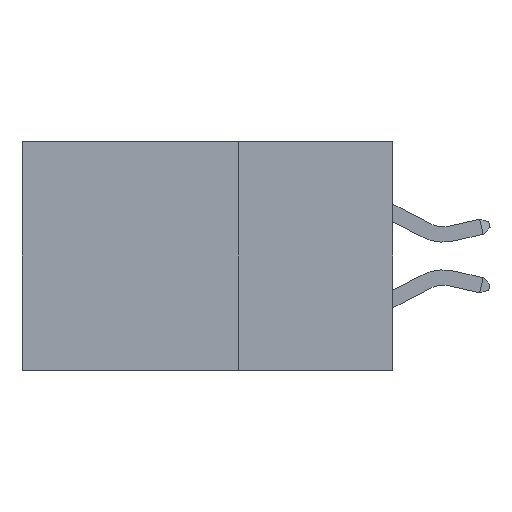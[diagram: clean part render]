
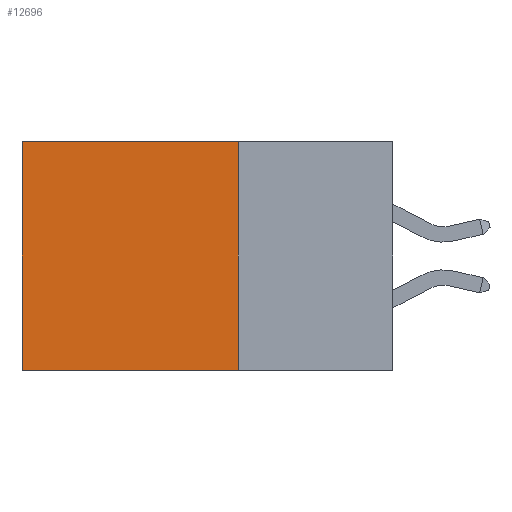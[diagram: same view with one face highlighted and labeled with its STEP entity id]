
A CAD part, left-side view. The second image highlights one B-rep face of the part: STEP entity #12696.
In plain terms, the highlighted planar face has unit normal (-1, 0, 0).
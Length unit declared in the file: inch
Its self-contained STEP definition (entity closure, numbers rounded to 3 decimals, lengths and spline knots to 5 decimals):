
#2719 = AXIS2_PLACEMENT_3D ( 'NONE', #17160, #15064, #10390 ) ;
#3897 = ORIENTED_EDGE ( 'NONE', *, *, #13775, .T. ) ;
#4847 = EDGE_LOOP ( 'NONE', ( #3897, #8581, #10344, #21569 ) ) ;
#4939 = LINE ( 'NONE', #21337, #16211 ) ;
#5085 = DIRECTION ( 'NONE',  ( 0., 1., 0. ) ) ;
#6063 = CARTESIAN_POINT ( 'NONE',  ( 0.2875, 0.6, -0.37 ) ) ;
#6627 = VECTOR ( 'NONE', #10901, 39.37008 ) ;
#7190 = DIRECTION ( 'NONE',  ( 0., 0., -1. ) ) ;
#8581 = ORIENTED_EDGE ( 'NONE', *, *, #19169, .F. ) ;
#10344 = ORIENTED_EDGE ( 'NONE', *, *, #15902, .F. ) ;
#10390 = DIRECTION ( 'NONE',  ( 0., 0., -1. ) ) ;
#10427 = CARTESIAN_POINT ( 'NONE',  ( 0.2875, 0.25, -0.37 ) ) ;
#10861 = VECTOR ( 'NONE', #7190, 39.37008 ) ;
#10901 = DIRECTION ( 'NONE',  ( 0., 0., -1. ) ) ;
#11781 = DIRECTION ( 'NONE',  ( 0., 1., 0. ) ) ;
#12696 = ADVANCED_FACE ( 'NONE', ( #29035 ), #24222, .F. ) ;
#13203 = CARTESIAN_POINT ( 'NONE',  ( 0.2875, 0.6, 0. ) ) ;
#13775 = EDGE_CURVE ( 'NONE', #26347, #25376, #20081, .T. ) ;
#15064 = DIRECTION ( 'NONE',  ( 1., 0., 0. ) ) ;
#15453 = VECTOR ( 'NONE', #11781, 39.37008 ) ;
#15463 = CARTESIAN_POINT ( 'NONE',  ( 0.2875, 0.25, 0. ) ) ;
#15902 = EDGE_CURVE ( 'NONE', #19752, #25351, #25389, .T. ) ;
#16211 = VECTOR ( 'NONE', #5085, 39.37008 ) ;
#17160 = CARTESIAN_POINT ( 'NONE',  ( 0.2875, 0.25, 0. ) ) ;
#18846 = CARTESIAN_POINT ( 'NONE',  ( 0.2875, 0.25, 0. ) ) ;
#19169 = EDGE_CURVE ( 'NONE', #25351, #25376, #4939, .T. ) ;
#19752 = VERTEX_POINT ( 'NONE', #15463 ) ;
#20081 = LINE ( 'NONE', #22489, #6627 ) ;
#21337 = CARTESIAN_POINT ( 'NONE',  ( 0.2875, 0.25, -0.37 ) ) ;
#21569 = ORIENTED_EDGE ( 'NONE', *, *, #25258, .T. ) ;
#22489 = CARTESIAN_POINT ( 'NONE',  ( 0.2875, 0.6, 0. ) ) ;
#24222 = PLANE ( 'NONE',  #2719 ) ;
#25258 = EDGE_CURVE ( 'NONE', #19752, #26347, #27728, .T. ) ;
#25351 = VERTEX_POINT ( 'NONE', #10427 ) ;
#25376 = VERTEX_POINT ( 'NONE', #6063 ) ;
#25389 = LINE ( 'NONE', #25535, #10861 ) ;
#25535 = CARTESIAN_POINT ( 'NONE',  ( 0.2875, 0.25, 0. ) ) ;
#26347 = VERTEX_POINT ( 'NONE', #13203 ) ;
#27728 = LINE ( 'NONE', #18846, #15453 ) ;
#29035 = FACE_OUTER_BOUND ( 'NONE', #4847, .T. ) ;
